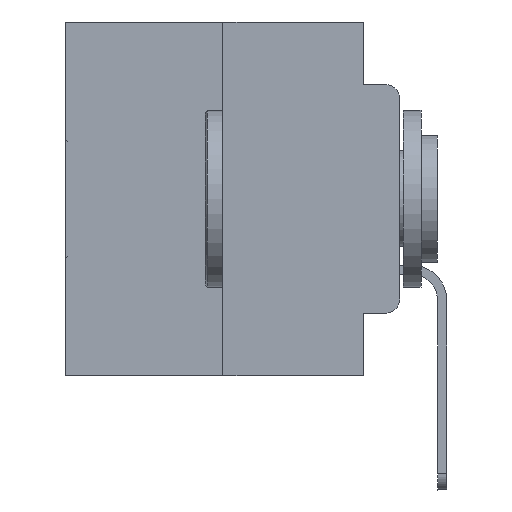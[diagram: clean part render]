
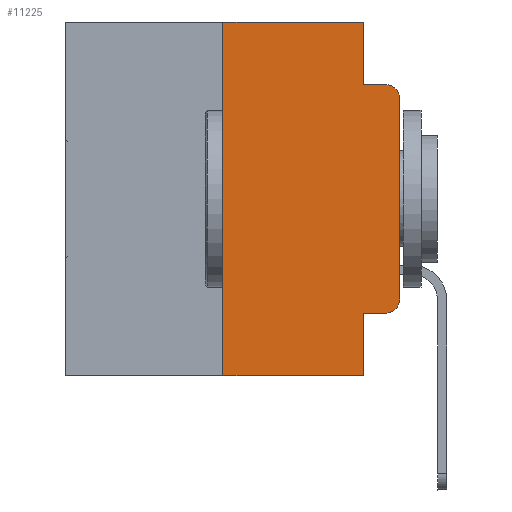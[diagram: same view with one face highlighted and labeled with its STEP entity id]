
A CAD part, left-side view. The second image highlights one B-rep face of the part: STEP entity #11225.
In plain terms, the highlighted planar face has unit normal (-1, 0, 0).
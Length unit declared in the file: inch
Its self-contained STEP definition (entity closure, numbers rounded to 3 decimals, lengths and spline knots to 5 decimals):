
#37 = VECTOR ( 'NONE', #4515, 39.37008 ) ;
#51 = CARTESIAN_POINT ( 'NONE',  ( 0., 0.02, -0.0885 ) ) ;
#378 = DIRECTION ( 'NONE',  ( 0., 0., -1. ) ) ;
#748 = DIRECTION ( 'NONE',  ( 0., 0., -1. ) ) ;
#1356 = EDGE_CURVE ( 'NONE', #25229, #1743, #2920, .T. ) ;
#1743 = VERTEX_POINT ( 'NONE', #14502 ) ;
#1967 = VERTEX_POINT ( 'NONE', #21922 ) ;
#1983 = CARTESIAN_POINT ( 'NONE',  ( 0., 0.051, 0. ) ) ;
#2920 = LINE ( 'NONE', #25906, #17329 ) ;
#2989 = CARTESIAN_POINT ( 'NONE',  ( 0., 0.473, -0.5 ) ) ;
#3144 = AXIS2_PLACEMENT_3D ( 'NONE', #24359, #27217, #10454 ) ;
#3734 = CARTESIAN_POINT ( 'NONE',  ( 0., 0., 0. ) ) ;
#4515 = DIRECTION ( 'NONE',  ( 0., -1., 0. ) ) ;
#5677 = CARTESIAN_POINT ( 'NONE',  ( 0., 0.25, 0. ) ) ;
#5866 = ORIENTED_EDGE ( 'NONE', *, *, #18013, .T. ) ;
#5885 = CARTESIAN_POINT ( 'NONE',  ( 0., 0.473, 0. ) ) ;
#5944 = VECTOR ( 'NONE', #26063, 39.37008 ) ;
#6477 = DIRECTION ( 'NONE',  ( 0., 0., -1. ) ) ;
#6924 = CARTESIAN_POINT ( 'NONE',  ( 0., 0.051, -0.4115 ) ) ;
#7664 = ORIENTED_EDGE ( 'NONE', *, *, #18201, .T. ) ;
#7828 = LINE ( 'NONE', #21725, #18665 ) ;
#8012 = EDGE_LOOP ( 'NONE', ( #7664, #12104, #11960, #23021, #18417, #29450, #20675, #29444, #5866, #15597 ) ) ;
#8236 = VECTOR ( 'NONE', #15521, 39.37008 ) ;
#8507 = EDGE_CURVE ( 'NONE', #12160, #18583, #21265, .T. ) ;
#8721 = FACE_OUTER_BOUND ( 'NONE', #8012, .T. ) ;
#9800 = EDGE_CURVE ( 'NONE', #15511, #18583, #7828, .T. ) ;
#10426 = LINE ( 'NONE', #5885, #8236 ) ;
#10454 = DIRECTION ( 'NONE',  ( 0., 0., -1. ) ) ;
#10890 = VECTOR ( 'NONE', #14451, 39.37008 ) ;
#11142 = DIRECTION ( 'NONE',  ( 0., 0., -1. ) ) ;
#11225 = ADVANCED_FACE ( 'NONE', ( #8721 ), #11290, .F. ) ;
#11290 = PLANE ( 'NONE',  #15825 ) ;
#11304 = LINE ( 'NONE', #6924, #37 ) ;
#11960 = ORIENTED_EDGE ( 'NONE', *, *, #26924, .F. ) ;
#12104 = ORIENTED_EDGE ( 'NONE', *, *, #23986, .T. ) ;
#12160 = VERTEX_POINT ( 'NONE', #29379 ) ;
#12827 = DIRECTION ( 'NONE',  ( 0., -1., 0. ) ) ;
#12999 = CARTESIAN_POINT ( 'NONE',  ( 0., 0.051, -0.4115 ) ) ;
#14451 = DIRECTION ( 'NONE',  ( 0., -1., 0. ) ) ;
#14472 = CARTESIAN_POINT ( 'NONE',  ( 0., 0., -0.3915 ) ) ;
#14502 = CARTESIAN_POINT ( 'NONE',  ( 0., 0.051, -0.0885 ) ) ;
#15332 = VERTEX_POINT ( 'NONE', #51 ) ;
#15375 = CARTESIAN_POINT ( 'NONE',  ( 0., 0.25, 0. ) ) ;
#15497 = VERTEX_POINT ( 'NONE', #25733 ) ;
#15511 = VERTEX_POINT ( 'NONE', #12999 ) ;
#15521 = DIRECTION ( 'NONE',  ( 0., -1., 0. ) ) ;
#15597 = ORIENTED_EDGE ( 'NONE', *, *, #25716, .T. ) ;
#15825 = AXIS2_PLACEMENT_3D ( 'NONE', #20511, #24462, #11142 ) ;
#16940 = VECTOR ( 'NONE', #29107, 39.37008 ) ;
#17329 = VECTOR ( 'NONE', #378, 39.37008 ) ;
#17652 = LINE ( 'NONE', #26883, #24712 ) ;
#17809 = VERTEX_POINT ( 'NONE', #15375 ) ;
#17877 = AXIS2_PLACEMENT_3D ( 'NONE', #17945, #27181, #6477 ) ;
#17881 = EDGE_CURVE ( 'NONE', #17809, #25229, #10426, .T. ) ;
#17945 = CARTESIAN_POINT ( 'NONE',  ( 0., 0.02, -0.3915 ) ) ;
#18013 = EDGE_CURVE ( 'NONE', #15511, #1967, #11304, .T. ) ;
#18201 = EDGE_CURVE ( 'NONE', #28238, #15497, #29257, .T. ) ;
#18417 = ORIENTED_EDGE ( 'NONE', *, *, #17881, .F. ) ;
#18583 = VERTEX_POINT ( 'NONE', #21936 ) ;
#18665 = VECTOR ( 'NONE', #748, 39.37008 ) ;
#19815 = CIRCLE ( 'NONE', #17877, 0.02 ) ;
#20511 = CARTESIAN_POINT ( 'NONE',  ( 0., 0.473, 0. ) ) ;
#20675 = ORIENTED_EDGE ( 'NONE', *, *, #8507, .T. ) ;
#21265 = LINE ( 'NONE', #2989, #10890 ) ;
#21725 = CARTESIAN_POINT ( 'NONE',  ( 0., 0.051, 0. ) ) ;
#21819 = LINE ( 'NONE', #5677, #5944 ) ;
#21922 = CARTESIAN_POINT ( 'NONE',  ( 0., 0.02, -0.4115 ) ) ;
#21936 = CARTESIAN_POINT ( 'NONE',  ( 0., 0.051, -0.5 ) ) ;
#23021 = ORIENTED_EDGE ( 'NONE', *, *, #1356, .F. ) ;
#23421 = CIRCLE ( 'NONE', #3144, 0.02 ) ;
#23986 = EDGE_CURVE ( 'NONE', #15497, #15332, #23421, .T. ) ;
#24359 = CARTESIAN_POINT ( 'NONE',  ( 0., 0.02, -0.1085 ) ) ;
#24462 = DIRECTION ( 'NONE',  ( 1., 0., 0. ) ) ;
#24712 = VECTOR ( 'NONE', #12827, 39.37008 ) ;
#25229 = VERTEX_POINT ( 'NONE', #1983 ) ;
#25716 = EDGE_CURVE ( 'NONE', #1967, #28238, #19815, .T. ) ;
#25733 = CARTESIAN_POINT ( 'NONE',  ( 0., 0., -0.1085 ) ) ;
#25906 = CARTESIAN_POINT ( 'NONE',  ( 0., 0.051, 0. ) ) ;
#26063 = DIRECTION ( 'NONE',  ( 0., 0., 1. ) ) ;
#26883 = CARTESIAN_POINT ( 'NONE',  ( 0., 0.051, -0.0885 ) ) ;
#26924 = EDGE_CURVE ( 'NONE', #1743, #15332, #17652, .T. ) ;
#27181 = DIRECTION ( 'NONE',  ( -1., 0., 0. ) ) ;
#27217 = DIRECTION ( 'NONE',  ( -1., 0., 0. ) ) ;
#28238 = VERTEX_POINT ( 'NONE', #14472 ) ;
#29107 = DIRECTION ( 'NONE',  ( 0., 0., 1. ) ) ;
#29257 = LINE ( 'NONE', #3734, #16940 ) ;
#29271 = EDGE_CURVE ( 'NONE', #12160, #17809, #21819, .T. ) ;
#29379 = CARTESIAN_POINT ( 'NONE',  ( 0., 0.25, -0.5 ) ) ;
#29444 = ORIENTED_EDGE ( 'NONE', *, *, #9800, .F. ) ;
#29450 = ORIENTED_EDGE ( 'NONE', *, *, #29271, .F. ) ;
